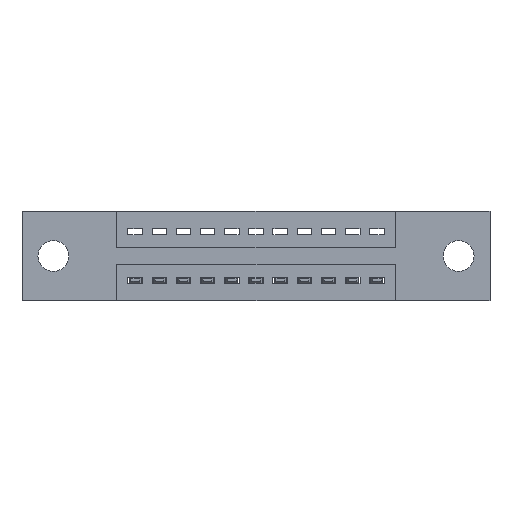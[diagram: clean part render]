
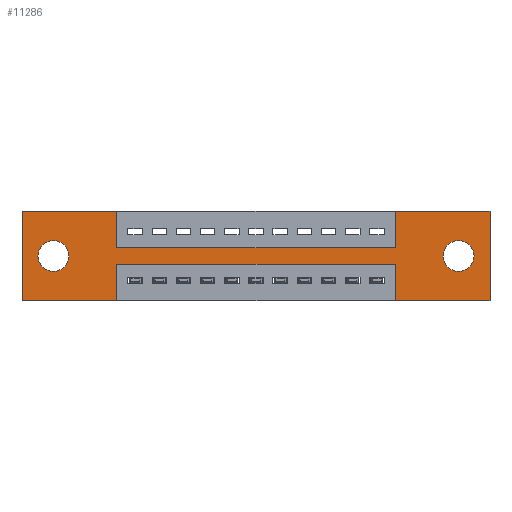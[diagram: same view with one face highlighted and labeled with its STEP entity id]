
A CAD part, front view. The second image highlights one B-rep face of the part: STEP entity #11286.
In plain terms, the highlighted planar face has unit normal (0, -1, 0).
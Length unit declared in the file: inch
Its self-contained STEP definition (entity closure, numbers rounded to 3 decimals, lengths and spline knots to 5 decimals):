
#197 = ORIENTED_EDGE ( 'NONE', *, *, #4840, .T. ) ;
#205 = VECTOR ( 'NONE', #11998, 39.37008 ) ;
#301 = ORIENTED_EDGE ( 'NONE', *, *, #1832, .T. ) ;
#581 = ORIENTED_EDGE ( 'NONE', *, *, #3560, .T. ) ;
#736 = ORIENTED_EDGE ( 'NONE', *, *, #7559, .T. ) ;
#767 = ORIENTED_EDGE ( 'NONE', *, *, #7601, .F. ) ;
#780 = AXIS2_PLACEMENT_3D ( 'NONE', #2368, #2366, #2355 ) ;
#812 = DIRECTION ( 'NONE',  ( 0., 0., 1. ) ) ;
#842 = CARTESIAN_POINT ( 'NONE',  ( 0.3925, 0., -0.15 ) ) ;
#869 = ORIENTED_EDGE ( 'NONE', *, *, #4707, .F. ) ;
#893 = ORIENTED_EDGE ( 'NONE', *, *, #12210, .F. ) ;
#919 = DIRECTION ( 'NONE',  ( 0., 0., -1. ) ) ;
#932 = CARTESIAN_POINT ( 'NONE',  ( 0.3925, 0., 0. ) ) ;
#1013 = CARTESIAN_POINT ( 'NONE',  ( 0.13, 0., -0.185 ) ) ;
#1052 = DIRECTION ( 'NONE',  ( 0., 0., -1. ) ) ;
#1069 = DIRECTION ( 'NONE',  ( 0., 1., 0. ) ) ;
#1108 = ORIENTED_EDGE ( 'NONE', *, *, #10225, .F. ) ;
#1149 = DIRECTION ( 'NONE',  ( 0., 1., 0. ) ) ;
#1210 = CARTESIAN_POINT ( 'NONE',  ( 1.805, 0., -0.185 ) ) ;
#1242 = CIRCLE ( 'NONE', #3422, 0.064 ) ;
#1359 = VERTEX_POINT ( 'NONE', #12273 ) ;
#1363 = ORIENTED_EDGE ( 'NONE', *, *, #4668, .F. ) ;
#1374 = ORIENTED_EDGE ( 'NONE', *, *, #12105, .F. ) ;
#1429 = FACE_BOUND ( 'NONE', #9804, .T. ) ;
#1455 = DIRECTION ( 'NONE',  ( 0., 0., 1. ) ) ;
#1526 = ORIENTED_EDGE ( 'NONE', *, *, #1905, .F. ) ;
#1529 = ORIENTED_EDGE ( 'NONE', *, *, #5397, .F. ) ;
#1546 = CARTESIAN_POINT ( 'NONE',  ( 1.5425, 0., 0. ) ) ;
#1660 = CARTESIAN_POINT ( 'NONE',  ( 1.935, 0., 0. ) ) ;
#1709 = ORIENTED_EDGE ( 'NONE', *, *, #3745, .F. ) ;
#1752 = FACE_BOUND ( 'NONE', #10200, .T. ) ;
#1831 = VERTEX_POINT ( 'NONE', #3807 ) ;
#1832 = EDGE_CURVE ( 'NONE', #2643, #3616, #1242, .T. ) ;
#1905 = EDGE_CURVE ( 'NONE', #8232, #6023, #5521, .T. ) ;
#1910 = ORIENTED_EDGE ( 'NONE', *, *, #5695, .F. ) ;
#1921 = ORIENTED_EDGE ( 'NONE', *, *, #6167, .F. ) ;
#1942 = ORIENTED_EDGE ( 'NONE', *, *, #8051, .F. ) ;
#1975 = AXIS2_PLACEMENT_3D ( 'NONE', #3277, #10749, #5232 ) ;
#2041 = VECTOR ( 'NONE', #11381, 39.37008 ) ;
#2114 = CARTESIAN_POINT ( 'NONE',  ( 1.805, 0., -0.121 ) ) ;
#2355 = DIRECTION ( 'NONE',  ( 0., 0., 1. ) ) ;
#2366 = DIRECTION ( 'NONE',  ( 0., 1., 0. ) ) ;
#2368 = CARTESIAN_POINT ( 'NONE',  ( 0.13, 0., -0.185 ) ) ;
#2385 = CARTESIAN_POINT ( 'NONE',  ( 0., 0., -0.37 ) ) ;
#2643 = VERTEX_POINT ( 'NONE', #8261 ) ;
#2876 = CARTESIAN_POINT ( 'NONE',  ( 0., 0., 0. ) ) ;
#2958 = CARTESIAN_POINT ( 'NONE',  ( 0., 0., -0.37 ) ) ;
#3049 = DIRECTION ( 'NONE',  ( 0., 0., -1. ) ) ;
#3083 = DIRECTION ( 'NONE',  ( 0., 1., 0. ) ) ;
#3123 = CARTESIAN_POINT ( 'NONE',  ( 1.805, 0., -0.185 ) ) ;
#3277 = CARTESIAN_POINT ( 'NONE',  ( 0., 0., -0.37 ) ) ;
#3394 = CARTESIAN_POINT ( 'NONE',  ( 1.935, 0., -0.37 ) ) ;
#3404 = VERTEX_POINT ( 'NONE', #3394 ) ;
#3422 = AXIS2_PLACEMENT_3D ( 'NONE', #3123, #3083, #3049 ) ;
#3560 = EDGE_CURVE ( 'NONE', #11431, #5834, #10769, .T. ) ;
#3598 = VECTOR ( 'NONE', #1455, 39.37008 ) ;
#3616 = VERTEX_POINT ( 'NONE', #2114 ) ;
#3624 = DIRECTION ( 'NONE',  ( -1., 0., 0. ) ) ;
#3653 = CARTESIAN_POINT ( 'NONE',  ( 0.3925, 0., -0.22 ) ) ;
#3745 = EDGE_CURVE ( 'NONE', #11562, #1831, #11175, .T. ) ;
#3807 = CARTESIAN_POINT ( 'NONE',  ( 0.3925, 0., -0.15 ) ) ;
#3886 = AXIS2_PLACEMENT_3D ( 'NONE', #1013, #1149, #812 ) ;
#3925 = LINE ( 'NONE', #9227, #6120 ) ;
#3940 = LINE ( 'NONE', #11734, #10993 ) ;
#4131 = CARTESIAN_POINT ( 'NONE',  ( 0., 0., 0. ) ) ;
#4284 = PLANE ( 'NONE',  #1975 ) ;
#4668 = EDGE_CURVE ( 'NONE', #4803, #3404, #8187, .T. ) ;
#4707 = EDGE_CURVE ( 'NONE', #7419, #7409, #7644, .T. ) ;
#4709 = CARTESIAN_POINT ( 'NONE',  ( 0.3925, 0., 0. ) ) ;
#4757 = VERTEX_POINT ( 'NONE', #2958 ) ;
#4803 = VERTEX_POINT ( 'NONE', #1660 ) ;
#4840 = EDGE_CURVE ( 'NONE', #3616, #2643, #6449, .T. ) ;
#4880 = CARTESIAN_POINT ( 'NONE',  ( 0., 0., -0.37 ) ) ;
#4974 = LINE ( 'NONE', #842, #205 ) ;
#4983 = CARTESIAN_POINT ( 'NONE',  ( 1.5425, 0., -0.37 ) ) ;
#5155 = CARTESIAN_POINT ( 'NONE',  ( 1.935, 0., 0. ) ) ;
#5221 = DIRECTION ( 'NONE',  ( 0., 0., -1. ) ) ;
#5232 = DIRECTION ( 'NONE',  ( 0., 0., -1. ) ) ;
#5397 = EDGE_CURVE ( 'NONE', #1831, #8232, #4974, .T. ) ;
#5419 = VECTOR ( 'NONE', #3624, 39.37008 ) ;
#5438 = CARTESIAN_POINT ( 'NONE',  ( 0.13, 0., -0.121 ) ) ;
#5521 = LINE ( 'NONE', #1546, #3598 ) ;
#5528 = CARTESIAN_POINT ( 'NONE',  ( 1.5425, 0., -0.15 ) ) ;
#5695 = EDGE_CURVE ( 'NONE', #8530, #11562, #3940, .T. ) ;
#5834 = VERTEX_POINT ( 'NONE', #8179 ) ;
#5882 = CARTESIAN_POINT ( 'NONE',  ( 1.5425, 0., -0.22 ) ) ;
#6023 = VERTEX_POINT ( 'NONE', #9623 ) ;
#6030 = LINE ( 'NONE', #4880, #7352 ) ;
#6120 = VECTOR ( 'NONE', #8602, 39.37008 ) ;
#6167 = EDGE_CURVE ( 'NONE', #4757, #8530, #3925, .T. ) ;
#6424 = LINE ( 'NONE', #2876, #8578 ) ;
#6449 = CIRCLE ( 'NONE', #10300, 0.064 ) ;
#6506 = VECTOR ( 'NONE', #8094, 39.37008 ) ;
#6678 = DIRECTION ( 'NONE',  ( 1., 0., 0. ) ) ;
#7352 = VECTOR ( 'NONE', #12122, 39.37008 ) ;
#7409 = VERTEX_POINT ( 'NONE', #11516 ) ;
#7419 = VERTEX_POINT ( 'NONE', #5882 ) ;
#7559 = EDGE_CURVE ( 'NONE', #5834, #11431, #9828, .T. ) ;
#7601 = EDGE_CURVE ( 'NONE', #7409, #1359, #7716, .T. ) ;
#7644 = LINE ( 'NONE', #3653, #5419 ) ;
#7716 = LINE ( 'NONE', #11506, #11615 ) ;
#7830 = EDGE_LOOP ( 'NONE', ( #767, #869, #893, #1108, #1363, #1374, #1526, #1529, #1709, #1910, #1921, #1942 ) ) ;
#7915 = VECTOR ( 'NONE', #5221, 39.37008 ) ;
#8051 = EDGE_CURVE ( 'NONE', #1359, #4757, #11604, .T. ) ;
#8094 = DIRECTION ( 'NONE',  ( -1., 0., 0. ) ) ;
#8179 = CARTESIAN_POINT ( 'NONE',  ( 0.13, 0., -0.249 ) ) ;
#8187 = LINE ( 'NONE', #5155, #7915 ) ;
#8232 = VERTEX_POINT ( 'NONE', #5528 ) ;
#8261 = CARTESIAN_POINT ( 'NONE',  ( 1.805, 0., -0.249 ) ) ;
#8387 = VERTEX_POINT ( 'NONE', #12155 ) ;
#8483 = VECTOR ( 'NONE', #919, 39.37008 ) ;
#8530 = VERTEX_POINT ( 'NONE', #4131 ) ;
#8578 = VECTOR ( 'NONE', #6678, 39.37008 ) ;
#8602 = DIRECTION ( 'NONE',  ( 0., 0., 1. ) ) ;
#8998 = FACE_OUTER_BOUND ( 'NONE', #7830, .T. ) ;
#9227 = CARTESIAN_POINT ( 'NONE',  ( 0., 0., 0. ) ) ;
#9623 = CARTESIAN_POINT ( 'NONE',  ( 1.5425, 0., 0. ) ) ;
#9804 = EDGE_LOOP ( 'NONE', ( #197, #301 ) ) ;
#9828 = CIRCLE ( 'NONE', #3886, 0.064 ) ;
#10200 = EDGE_LOOP ( 'NONE', ( #581, #736 ) ) ;
#10225 = EDGE_CURVE ( 'NONE', #3404, #8387, #6030, .T. ) ;
#10300 = AXIS2_PLACEMENT_3D ( 'NONE', #1210, #1069, #1052 ) ;
#10749 = DIRECTION ( 'NONE',  ( 0., -1., 0. ) ) ;
#10769 = CIRCLE ( 'NONE', #780, 0.064 ) ;
#10993 = VECTOR ( 'NONE', #11769, 39.37008 ) ;
#11175 = LINE ( 'NONE', #932, #8483 ) ;
#11224 = DIRECTION ( 'NONE',  ( 0., 0., -1. ) ) ;
#11286 = ADVANCED_FACE ( 'NONE', ( #1429, #1752, #8998 ), #4284, .T. ) ;
#11381 = DIRECTION ( 'NONE',  ( 0., 0., 1. ) ) ;
#11431 = VERTEX_POINT ( 'NONE', #5438 ) ;
#11506 = CARTESIAN_POINT ( 'NONE',  ( 0.3925, 0., -0.37 ) ) ;
#11516 = CARTESIAN_POINT ( 'NONE',  ( 0.3925, 0., -0.22 ) ) ;
#11562 = VERTEX_POINT ( 'NONE', #4709 ) ;
#11604 = LINE ( 'NONE', #2385, #6506 ) ;
#11615 = VECTOR ( 'NONE', #11224, 39.37008 ) ;
#11654 = LINE ( 'NONE', #4983, #2041 ) ;
#11734 = CARTESIAN_POINT ( 'NONE',  ( 0., 0., 0. ) ) ;
#11769 = DIRECTION ( 'NONE',  ( 1., 0., 0. ) ) ;
#11998 = DIRECTION ( 'NONE',  ( 1., 0., 0. ) ) ;
#12105 = EDGE_CURVE ( 'NONE', #6023, #4803, #6424, .T. ) ;
#12122 = DIRECTION ( 'NONE',  ( -1., 0., 0. ) ) ;
#12155 = CARTESIAN_POINT ( 'NONE',  ( 1.5425, 0., -0.37 ) ) ;
#12210 = EDGE_CURVE ( 'NONE', #8387, #7419, #11654, .T. ) ;
#12273 = CARTESIAN_POINT ( 'NONE',  ( 0.3925, 0., -0.37 ) ) ;
